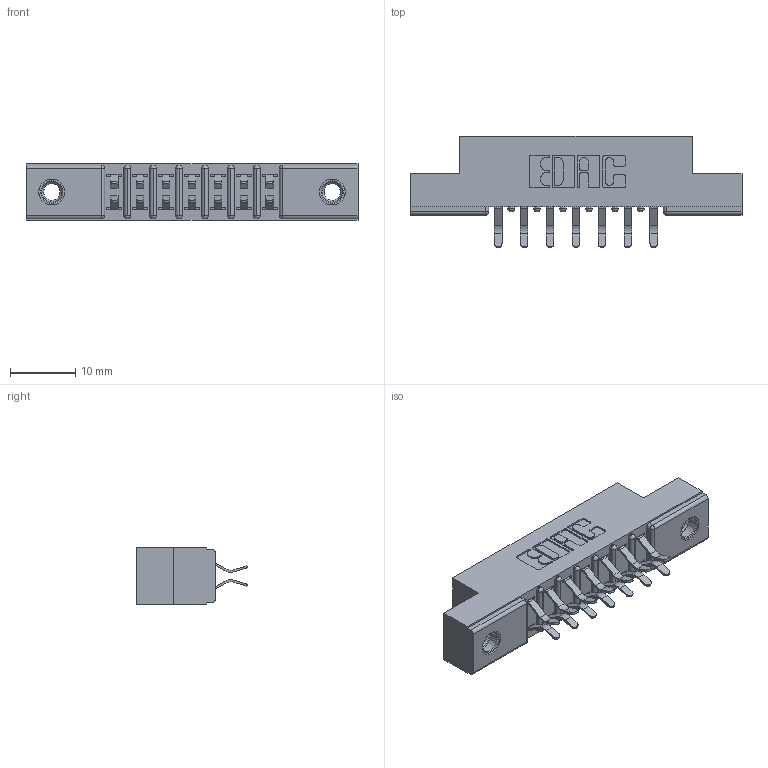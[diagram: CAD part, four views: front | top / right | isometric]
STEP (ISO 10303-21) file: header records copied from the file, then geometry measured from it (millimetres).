
FILE_DESCRIPTION (( 'STEP AP203' ), '1' );
FILE_NAME ('307-014-556-207.STEP', '2019-09-05T18:50:06', ( '' ), ( '' ), 'SwSTEP 2.0', 'SolidWorks 2016', '' );
FILE_SCHEMA (( 'CONFIG_CONTROL_DESIGN' ));
Length unit declared in the file: inch
Products named in the file (4): 307 Part_.156 Dia Mounting Holes; 307-290-001_556; 307-014-556-207; 345-250-001_345-250-005-103
Assembly tree (17 placements, depth 2):
  307-014-556-207
    307 Part_.156 Dia Mounting Holes
    307-290-001_556  x14
    345-250-001_345-250-005-103  x2
Bounding box: 50.75 x 16.97 x 8.71 mm (x, y, z)
Volume: 3305.2 mm3; surface area: 5079.6 mm2
Topology: 17 solids, 17 shells, 886 faces, 2447 edges, 1582 vertices
Faces by surface type: plane 564, cylinder 290, sphere 16, cone 12, torus 4
Entity records: 11829 total; most frequent: CARTESIAN_POINT 1930, DIRECTION 1915, ORIENTED_EDGE 1902, EDGE_CURVE 951, VECTOR 713, LINE 713, VERTEX_POINT 616, AXIS2_PLACEMENT_3D 601
